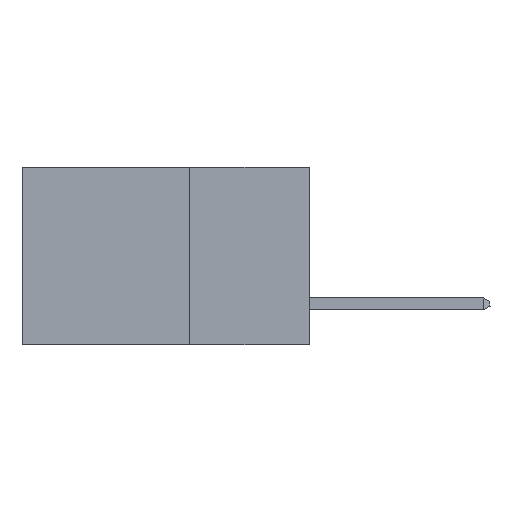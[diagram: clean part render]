
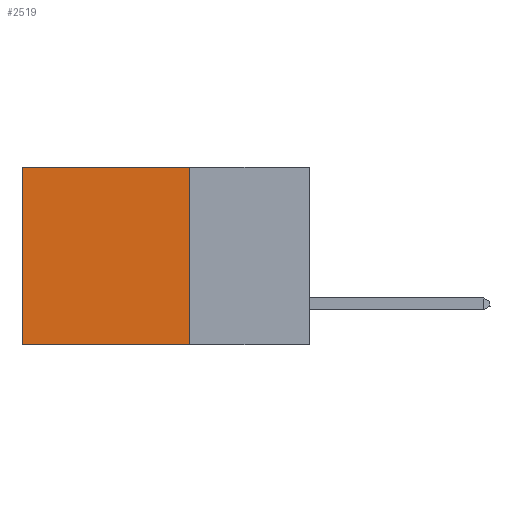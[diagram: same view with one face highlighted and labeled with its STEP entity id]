
A CAD part, left-side view. The second image highlights one B-rep face of the part: STEP entity #2519.
In plain terms, the highlighted planar face has unit normal (-1, 0, 0).
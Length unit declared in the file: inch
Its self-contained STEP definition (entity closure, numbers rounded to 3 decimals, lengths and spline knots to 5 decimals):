
#1 = VECTOR ( 'NONE', #29114, 39.37008 ) ;
#2519 = ADVANCED_FACE ( 'NONE', ( #18703 ), #9377, .F. ) ;
#2600 = DIRECTION ( 'NONE',  ( 0., 0., -1. ) ) ;
#2918 = LINE ( 'NONE', #15855, #37065 ) ;
#3021 = DIRECTION ( 'NONE',  ( 1., 0., 0. ) ) ;
#3454 = EDGE_CURVE ( 'NONE', #40703, #9112, #2918, .T. ) ;
#8464 = VECTOR ( 'NONE', #20242, 39.37008 ) ;
#9112 = VERTEX_POINT ( 'NONE', #35003 ) ;
#9377 = PLANE ( 'NONE',  #22655 ) ;
#11187 = EDGE_CURVE ( 'NONE', #19384, #9112, #11986, .T. ) ;
#11685 = CARTESIAN_POINT ( 'NONE',  ( 0.2875, 0.25, 0. ) ) ;
#11986 = LINE ( 'NONE', #27907, #37443 ) ;
#14752 = DIRECTION ( 'NONE',  ( 0., 1., 0. ) ) ;
#14888 = LINE ( 'NONE', #40791, #8464 ) ;
#15855 = CARTESIAN_POINT ( 'NONE',  ( 0.2875, 0.6, 0. ) ) ;
#16182 = CARTESIAN_POINT ( 'NONE',  ( 0.2875, 0.25, 0. ) ) ;
#17689 = EDGE_CURVE ( 'NONE', #31522, #19384, #38904, .T. ) ;
#18193 = EDGE_LOOP ( 'NONE', ( #36922, #29103, #31486, #20236 ) ) ;
#18689 = CARTESIAN_POINT ( 'NONE',  ( 0.2875, 0.25, -0.37 ) ) ;
#18703 = FACE_OUTER_BOUND ( 'NONE', #18193, .T. ) ;
#19384 = VERTEX_POINT ( 'NONE', #18689 ) ;
#20236 = ORIENTED_EDGE ( 'NONE', *, *, #32981, .T. ) ;
#20242 = DIRECTION ( 'NONE',  ( 0., 1., 0. ) ) ;
#22655 = AXIS2_PLACEMENT_3D ( 'NONE', #31665, #3021, #2600 ) ;
#27563 = CARTESIAN_POINT ( 'NONE',  ( 0.2875, 0.6, 0. ) ) ;
#27907 = CARTESIAN_POINT ( 'NONE',  ( 0.2875, 0.25, -0.37 ) ) ;
#29103 = ORIENTED_EDGE ( 'NONE', *, *, #11187, .F. ) ;
#29114 = DIRECTION ( 'NONE',  ( 0., 0., -1. ) ) ;
#31486 = ORIENTED_EDGE ( 'NONE', *, *, #17689, .F. ) ;
#31522 = VERTEX_POINT ( 'NONE', #11685 ) ;
#31665 = CARTESIAN_POINT ( 'NONE',  ( 0.2875, 0.25, 0. ) ) ;
#32981 = EDGE_CURVE ( 'NONE', #31522, #40703, #14888, .T. ) ;
#35003 = CARTESIAN_POINT ( 'NONE',  ( 0.2875, 0.6, -0.37 ) ) ;
#36922 = ORIENTED_EDGE ( 'NONE', *, *, #3454, .T. ) ;
#37065 = VECTOR ( 'NONE', #41762, 39.37008 ) ;
#37443 = VECTOR ( 'NONE', #14752, 39.37008 ) ;
#38904 = LINE ( 'NONE', #16182, #1 ) ;
#40703 = VERTEX_POINT ( 'NONE', #27563 ) ;
#40791 = CARTESIAN_POINT ( 'NONE',  ( 0.2875, 0.25, 0. ) ) ;
#41762 = DIRECTION ( 'NONE',  ( 0., 0., -1. ) ) ;
